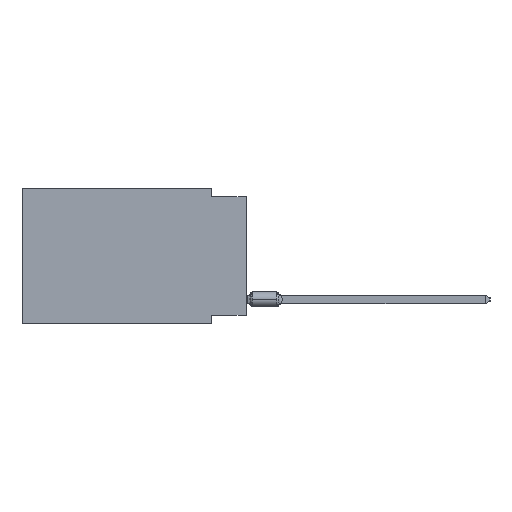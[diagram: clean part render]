
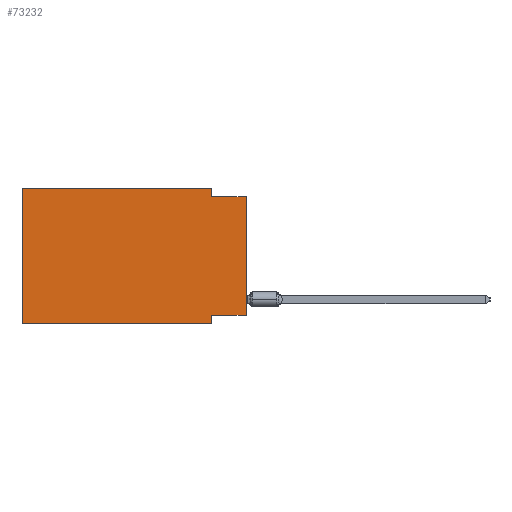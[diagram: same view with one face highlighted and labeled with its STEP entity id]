
A CAD part, left-side view. The second image highlights one B-rep face of the part: STEP entity #73232.
In plain terms, the highlighted planar face has unit normal (-1, 0, 0).
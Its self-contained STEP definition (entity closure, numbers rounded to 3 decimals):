
#1386 = CARTESIAN_POINT ( 'NONE',  ( 0., 2.54, -0.635 ) ) ;
#1707 = VERTEX_POINT ( 'NONE', #1386 ) ;
#2157 = ORIENTED_EDGE ( 'NONE', *, *, #49121, .T. ) ;
#3399 = DIRECTION ( 'NONE',  ( 0., 0., 1. ) ) ;
#3426 = DIRECTION ( 'NONE',  ( 0., 0., -1. ) ) ;
#4651 = VECTOR ( 'NONE', #23117, 1000. ) ;
#4845 = ORIENTED_EDGE ( 'NONE', *, *, #29861, .F. ) ;
#5308 = EDGE_CURVE ( 'NONE', #1707, #5525, #29481, .T. ) ;
#5525 = VERTEX_POINT ( 'NONE', #27780 ) ;
#6466 = LINE ( 'NONE', #6858, #24789 ) ;
#6858 = CARTESIAN_POINT ( 'NONE',  ( 0., 0., 0. ) ) ;
#8123 = ORIENTED_EDGE ( 'NONE', *, *, #78488, .T. ) ;
#9574 = CARTESIAN_POINT ( 'NONE',  ( 0., 16.383, 0. ) ) ;
#9683 = VERTEX_POINT ( 'NONE', #51531 ) ;
#10445 = VERTEX_POINT ( 'NONE', #39021 ) ;
#10577 = DIRECTION ( 'NONE',  ( 0., -1., 0. ) ) ;
#12178 = CARTESIAN_POINT ( 'NONE',  ( 0., 2.54, -9.271 ) ) ;
#12883 = DIRECTION ( 'NONE',  ( 0., 1., 0. ) ) ;
#12932 = CARTESIAN_POINT ( 'NONE',  ( 0., 2.54, -9.906 ) ) ;
#14833 = VECTOR ( 'NONE', #12883, 1000. ) ;
#14978 = CARTESIAN_POINT ( 'NONE',  ( 0., 2.54, 0. ) ) ;
#15154 = ORIENTED_EDGE ( 'NONE', *, *, #69333, .F. ) ;
#19486 = FACE_OUTER_BOUND ( 'NONE', #20808, .T. ) ;
#20808 = EDGE_LOOP ( 'NONE', ( #2157, #29460, #15154, #23233, #58976, #8123, #62139, #4845 ) ) ;
#22241 = VECTOR ( 'NONE', #76212, 1000. ) ;
#23117 = DIRECTION ( 'NONE',  ( 0., -1., 0. ) ) ;
#23233 = ORIENTED_EDGE ( 'NONE', *, *, #26678, .F. ) ;
#24789 = VECTOR ( 'NONE', #39326, 1000. ) ;
#26678 = EDGE_CURVE ( 'NONE', #10445, #39335, #65565, .T. ) ;
#27780 = CARTESIAN_POINT ( 'NONE',  ( 0., 0., -0.635 ) ) ;
#29057 = VERTEX_POINT ( 'NONE', #77563 ) ;
#29460 = ORIENTED_EDGE ( 'NONE', *, *, #5308, .F. ) ;
#29481 = LINE ( 'NONE', #60331, #51914 ) ;
#29861 = EDGE_CURVE ( 'NONE', #29057, #72670, #62633, .T. ) ;
#32215 = DIRECTION ( 'NONE',  ( 1., 0., 0. ) ) ;
#39021 = CARTESIAN_POINT ( 'NONE',  ( 0., 16.383, 0. ) ) ;
#39248 = VECTOR ( 'NONE', #3399, 1000. ) ;
#39326 = DIRECTION ( 'NONE',  ( 0., 0., 1. ) ) ;
#39335 = VERTEX_POINT ( 'NONE', #57544 ) ;
#46721 = VERTEX_POINT ( 'NONE', #67847 ) ;
#49020 = CARTESIAN_POINT ( 'NONE',  ( 0., 16.383, -9.906 ) ) ;
#49121 = EDGE_CURVE ( 'NONE', #29057, #5525, #6466, .T. ) ;
#49499 = EDGE_CURVE ( 'NONE', #72670, #46721, #69644, .T. ) ;
#51531 = CARTESIAN_POINT ( 'NONE',  ( 0., 16.383, -9.906 ) ) ;
#51914 = VECTOR ( 'NONE', #10577, 1000. ) ;
#52331 = PLANE ( 'NONE',  #79500 ) ;
#55460 = VECTOR ( 'NONE', #3426, 1000. ) ;
#57544 = CARTESIAN_POINT ( 'NONE',  ( 0., 2.54, 0. ) ) ;
#57802 = VECTOR ( 'NONE', #71721, 1000. ) ;
#58976 = ORIENTED_EDGE ( 'NONE', *, *, #65095, .F. ) ;
#60331 = CARTESIAN_POINT ( 'NONE',  ( 0., 0., -0.635 ) ) ;
#62139 = ORIENTED_EDGE ( 'NONE', *, *, #49499, .F. ) ;
#62633 = LINE ( 'NONE', #75362, #14833 ) ;
#63465 = CARTESIAN_POINT ( 'NONE',  ( 0., 16.383, 0. ) ) ;
#65095 = EDGE_CURVE ( 'NONE', #9683, #10445, #78610, .T. ) ;
#65565 = LINE ( 'NONE', #78283, #57802 ) ;
#67847 = CARTESIAN_POINT ( 'NONE',  ( 0., 2.54, -9.906 ) ) ;
#69333 = EDGE_CURVE ( 'NONE', #39335, #1707, #77850, .T. ) ;
#69644 = LINE ( 'NONE', #12932, #22241 ) ;
#71721 = DIRECTION ( 'NONE',  ( 0., -1., 0. ) ) ;
#72670 = VERTEX_POINT ( 'NONE', #12178 ) ;
#73232 = ADVANCED_FACE ( 'NONE', ( #19486 ), #52331, .F. ) ;
#74485 = LINE ( 'NONE', #49020, #4651 ) ;
#75362 = CARTESIAN_POINT ( 'NONE',  ( 0., 0., -9.271 ) ) ;
#76212 = DIRECTION ( 'NONE',  ( 0., 0., -1. ) ) ;
#77393 = DIRECTION ( 'NONE',  ( 0., 0., -1. ) ) ;
#77563 = CARTESIAN_POINT ( 'NONE',  ( 0., 0., -9.271 ) ) ;
#77850 = LINE ( 'NONE', #14978, #55460 ) ;
#78283 = CARTESIAN_POINT ( 'NONE',  ( 0., 16.383, 0. ) ) ;
#78488 = EDGE_CURVE ( 'NONE', #9683, #46721, #74485, .T. ) ;
#78610 = LINE ( 'NONE', #9574, #39248 ) ;
#79500 = AXIS2_PLACEMENT_3D ( 'NONE', #63465, #32215, #77393 ) ;
